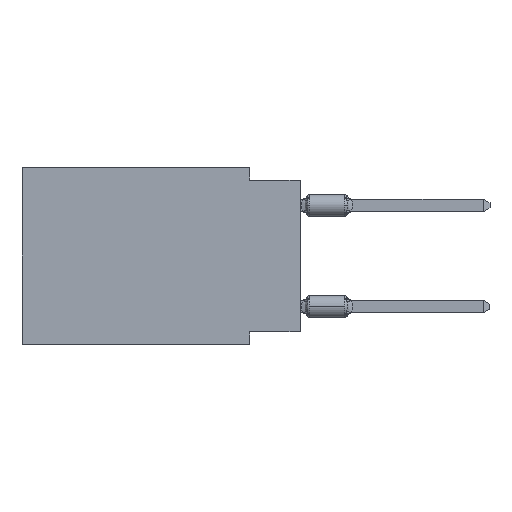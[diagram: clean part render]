
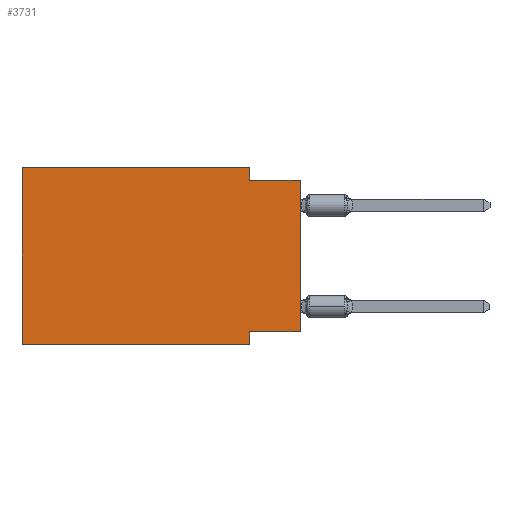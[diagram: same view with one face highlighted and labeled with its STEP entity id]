
A CAD part, left-side view. The second image highlights one B-rep face of the part: STEP entity #3731.
In plain terms, the highlighted planar face has unit normal (-1, 0, 0).
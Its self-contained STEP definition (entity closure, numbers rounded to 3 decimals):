
#428 = CARTESIAN_POINT ( 'NONE',  ( 0., 2.54, -0.635 ) ) ;
#598 = VERTEX_POINT ( 'NONE', #18314 ) ;
#735 = DIRECTION ( 'NONE',  ( 0., -1., 0. ) ) ;
#1450 = VERTEX_POINT ( 'NONE', #3223 ) ;
#1562 = ORIENTED_EDGE ( 'NONE', *, *, #9029, .F. ) ;
#1886 = EDGE_LOOP ( 'NONE', ( #20739, #1562, #22870, #9156, #11722, #18065, #16994, #9210 ) ) ;
#3223 = CARTESIAN_POINT ( 'NONE',  ( 0., 2.54, -8.255 ) ) ;
#3397 = DIRECTION ( 'NONE',  ( 0., 0., -1. ) ) ;
#3409 = VECTOR ( 'NONE', #18574, 1000. ) ;
#3460 = LINE ( 'NONE', #14766, #3409 ) ;
#3731 = ADVANCED_FACE ( 'NONE', ( #9869 ), #15520, .F. ) ;
#4318 = VERTEX_POINT ( 'NONE', #428 ) ;
#4397 = VERTEX_POINT ( 'NONE', #22909 ) ;
#4443 = EDGE_CURVE ( 'NONE', #17263, #1450, #18003, .T. ) ;
#5217 = VECTOR ( 'NONE', #8713, 1000. ) ;
#5272 = EDGE_CURVE ( 'NONE', #9936, #10170, #13884, .T. ) ;
#5339 = LINE ( 'NONE', #12957, #5217 ) ;
#5904 = EDGE_CURVE ( 'NONE', #4397, #9936, #5339, .T. ) ;
#6185 = DIRECTION ( 'NONE',  ( 1., 0., 0. ) ) ;
#6522 = CARTESIAN_POINT ( 'NONE',  ( 0., 13.97, 0. ) ) ;
#6845 = LINE ( 'NONE', #21823, #14273 ) ;
#6859 = LINE ( 'NONE', #20354, #16310 ) ;
#8713 = DIRECTION ( 'NONE',  ( 0., 0., 1. ) ) ;
#9029 = EDGE_CURVE ( 'NONE', #4318, #17221, #6845, .T. ) ;
#9151 = EDGE_CURVE ( 'NONE', #1450, #598, #14588, .T. ) ;
#9156 = ORIENTED_EDGE ( 'NONE', *, *, #5272, .F. ) ;
#9210 = ORIENTED_EDGE ( 'NONE', *, *, #4443, .F. ) ;
#9417 = DIRECTION ( 'NONE',  ( 0., 0., -1. ) ) ;
#9869 = FACE_OUTER_BOUND ( 'NONE', #1886, .T. ) ;
#9936 = VERTEX_POINT ( 'NONE', #23851 ) ;
#10017 = VECTOR ( 'NONE', #19609, 1000. ) ;
#10170 = VERTEX_POINT ( 'NONE', #11555 ) ;
#10268 = CARTESIAN_POINT ( 'NONE',  ( 0., 0., -8.255 ) ) ;
#10300 = CARTESIAN_POINT ( 'NONE',  ( 0., 0., -8.255 ) ) ;
#10528 = LINE ( 'NONE', #12114, #10017 ) ;
#10692 = VECTOR ( 'NONE', #735, 1000. ) ;
#11131 = CARTESIAN_POINT ( 'NONE',  ( 0., 2.54, -8.89 ) ) ;
#11290 = EDGE_CURVE ( 'NONE', #4397, #598, #3460, .T. ) ;
#11555 = CARTESIAN_POINT ( 'NONE',  ( 0., 2.54, 0. ) ) ;
#11722 = ORIENTED_EDGE ( 'NONE', *, *, #5904, .F. ) ;
#12114 = CARTESIAN_POINT ( 'NONE',  ( 0., 0., 0. ) ) ;
#12497 = DIRECTION ( 'NONE',  ( 0., -1., 0. ) ) ;
#12957 = CARTESIAN_POINT ( 'NONE',  ( 0., 13.97, 0. ) ) ;
#13663 = DIRECTION ( 'NONE',  ( 0., 0., -1. ) ) ;
#13884 = LINE ( 'NONE', #6522, #10692 ) ;
#14180 = VECTOR ( 'NONE', #15922, 1000. ) ;
#14273 = VECTOR ( 'NONE', #12497, 1000. ) ;
#14588 = LINE ( 'NONE', #11131, #17033 ) ;
#14766 = CARTESIAN_POINT ( 'NONE',  ( 0., 13.97, -8.89 ) ) ;
#15520 = PLANE ( 'NONE',  #18482 ) ;
#15922 = DIRECTION ( 'NONE',  ( 0., 1., 0. ) ) ;
#16078 = CARTESIAN_POINT ( 'NONE',  ( 0., 0., -0.635 ) ) ;
#16310 = VECTOR ( 'NONE', #3397, 1000. ) ;
#16994 = ORIENTED_EDGE ( 'NONE', *, *, #9151, .F. ) ;
#17033 = VECTOR ( 'NONE', #9417, 1000. ) ;
#17221 = VERTEX_POINT ( 'NONE', #16078 ) ;
#17263 = VERTEX_POINT ( 'NONE', #10300 ) ;
#18003 = LINE ( 'NONE', #10268, #14180 ) ;
#18065 = ORIENTED_EDGE ( 'NONE', *, *, #11290, .T. ) ;
#18314 = CARTESIAN_POINT ( 'NONE',  ( 0., 2.54, -8.89 ) ) ;
#18482 = AXIS2_PLACEMENT_3D ( 'NONE', #23002, #6185, #13663 ) ;
#18574 = DIRECTION ( 'NONE',  ( 0., -1., 0. ) ) ;
#19609 = DIRECTION ( 'NONE',  ( 0., 0., 1. ) ) ;
#19742 = EDGE_CURVE ( 'NONE', #10170, #4318, #6859, .T. ) ;
#20354 = CARTESIAN_POINT ( 'NONE',  ( 0., 2.54, 0. ) ) ;
#20739 = ORIENTED_EDGE ( 'NONE', *, *, #21182, .T. ) ;
#21182 = EDGE_CURVE ( 'NONE', #17263, #17221, #10528, .T. ) ;
#21823 = CARTESIAN_POINT ( 'NONE',  ( 0., 0., -0.635 ) ) ;
#22870 = ORIENTED_EDGE ( 'NONE', *, *, #19742, .F. ) ;
#22909 = CARTESIAN_POINT ( 'NONE',  ( 0., 13.97, -8.89 ) ) ;
#23002 = CARTESIAN_POINT ( 'NONE',  ( 0., 13.97, 0. ) ) ;
#23851 = CARTESIAN_POINT ( 'NONE',  ( 0., 13.97, 0. ) ) ;
